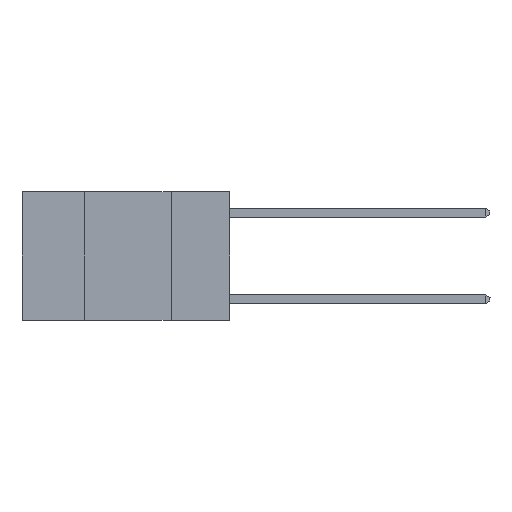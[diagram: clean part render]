
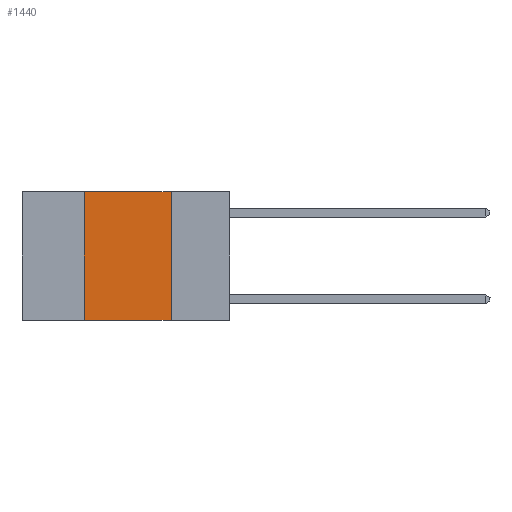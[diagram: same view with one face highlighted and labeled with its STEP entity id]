
A CAD part, left-side view. The second image highlights one B-rep face of the part: STEP entity #1440.
In plain terms, the highlighted planar face has unit normal (-1, 0, 0).
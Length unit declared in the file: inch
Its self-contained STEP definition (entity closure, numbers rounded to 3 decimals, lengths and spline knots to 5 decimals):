
#11 = FACE_OUTER_BOUND ( 'NONE', #5595, .T. ) ;
#203 = PLANE ( 'NONE',  #1235 ) ;
#220 = DIRECTION ( 'NONE',  ( 1., 0., 0. ) ) ;
#847 = VECTOR ( 'NONE', #8956, 39.37008 ) ;
#1023 = EDGE_CURVE ( 'NONE', #5400, #7212, #2605, .T. ) ;
#1082 = EDGE_CURVE ( 'NONE', #7202, #3447, #3791, .T. ) ;
#1097 = EDGE_CURVE ( 'NONE', #7202, #7212, #7297, .T. ) ;
#1235 = AXIS2_PLACEMENT_3D ( 'NONE', #8815, #220, #2437 ) ;
#1440 = ADVANCED_FACE ( 'NONE', ( #11 ), #203, .F. ) ;
#2369 = DIRECTION ( 'NONE',  ( 0., 0., 1. ) ) ;
#2437 = DIRECTION ( 'NONE',  ( 0., 0., -1. ) ) ;
#2476 = LINE ( 'NONE', #6716, #7087 ) ;
#2605 = LINE ( 'NONE', #5563, #4793 ) ;
#3241 = ORIENTED_EDGE ( 'NONE', *, *, #1097, .T. ) ;
#3393 = CARTESIAN_POINT ( 'NONE',  ( 0., 0.17, -0.37 ) ) ;
#3447 = VERTEX_POINT ( 'NONE', #6759 ) ;
#3539 = DIRECTION ( 'NONE',  ( 0., 0., -1. ) ) ;
#3637 = EDGE_CURVE ( 'NONE', #3447, #5400, #2476, .T. ) ;
#3791 = LINE ( 'NONE', #6087, #9459 ) ;
#4793 = VECTOR ( 'NONE', #3539, 39.37008 ) ;
#5125 = ORIENTED_EDGE ( 'NONE', *, *, #1023, .F. ) ;
#5164 = CARTESIAN_POINT ( 'NONE',  ( 0., 0.17, 0. ) ) ;
#5400 = VERTEX_POINT ( 'NONE', #5164 ) ;
#5563 = CARTESIAN_POINT ( 'NONE',  ( 0., 0.17, 0. ) ) ;
#5595 = EDGE_LOOP ( 'NONE', ( #5125, #7053, #5596, #3241 ) ) ;
#5596 = ORIENTED_EDGE ( 'NONE', *, *, #1082, .F. ) ;
#6087 = CARTESIAN_POINT ( 'NONE',  ( 0., 0.42, 0. ) ) ;
#6451 = CARTESIAN_POINT ( 'NONE',  ( 0., 0.42, -0.37 ) ) ;
#6716 = CARTESIAN_POINT ( 'NONE',  ( 0., 0.6, 0. ) ) ;
#6759 = CARTESIAN_POINT ( 'NONE',  ( 0., 0.42, 0. ) ) ;
#7053 = ORIENTED_EDGE ( 'NONE', *, *, #3637, .F. ) ;
#7087 = VECTOR ( 'NONE', #9591, 39.37008 ) ;
#7202 = VERTEX_POINT ( 'NONE', #6451 ) ;
#7212 = VERTEX_POINT ( 'NONE', #3393 ) ;
#7297 = LINE ( 'NONE', #10181, #847 ) ;
#8815 = CARTESIAN_POINT ( 'NONE',  ( 0., 0.6, 0. ) ) ;
#8956 = DIRECTION ( 'NONE',  ( 0., -1., 0. ) ) ;
#9459 = VECTOR ( 'NONE', #2369, 39.37008 ) ;
#9591 = DIRECTION ( 'NONE',  ( 0., -1., 0. ) ) ;
#10181 = CARTESIAN_POINT ( 'NONE',  ( 0., 0.6, -0.37 ) ) ;
